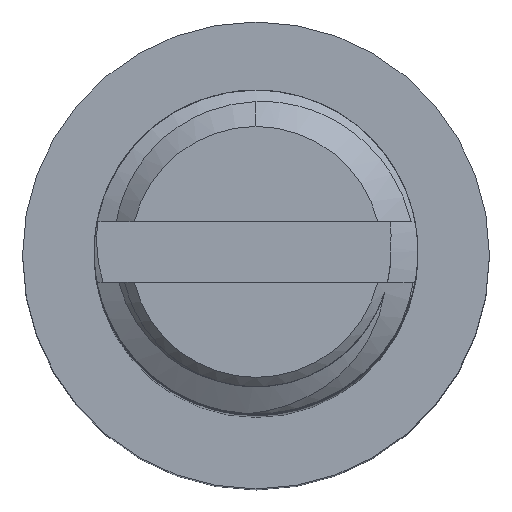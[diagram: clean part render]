
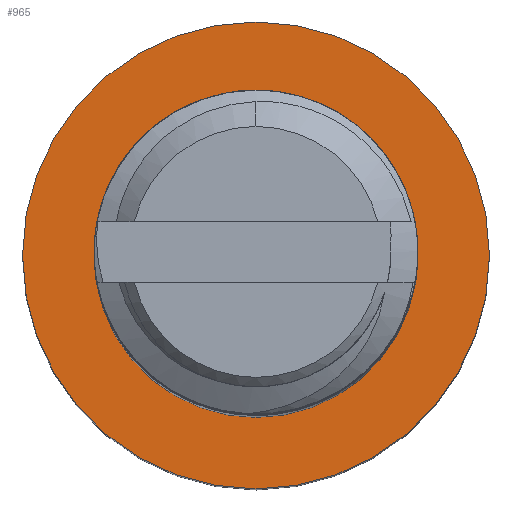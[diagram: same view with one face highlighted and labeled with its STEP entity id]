
A CAD part, top view. The second image highlights one B-rep face of the part: STEP entity #965.
In plain terms, the highlighted planar face has unit normal (0, 0, 1).
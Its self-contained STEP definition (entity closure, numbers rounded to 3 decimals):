
#155 = EDGE_CURVE ( 'NONE', #8737, #4906, #6477, .T. ) ;
#169 = ORIENTED_EDGE ( 'NONE', *, *, #5613, .F. ) ;
#965 = ADVANCED_FACE ( 'NONE', ( #6324, #4373 ), #6561, .T. ) ;
#1108 = CARTESIAN_POINT ( 'NONE',  ( 0., -2.705, -33.528 ) ) ;
#1222 = DIRECTION ( 'NONE',  ( 0., 0., 1. ) ) ;
#1231 = CIRCLE ( 'NONE', #2473, 2.705 ) ;
#1391 = CARTESIAN_POINT ( 'NONE',  ( 0., 0., -33.528 ) ) ;
#1468 = AXIS2_PLACEMENT_3D ( 'NONE', #5819, #2209, #7310 ) ;
#1597 = EDGE_LOOP ( 'NONE', ( #7868, #169 ) ) ;
#2125 = DIRECTION ( 'NONE',  ( 0., 1., 0. ) ) ;
#2209 = DIRECTION ( 'NONE',  ( 0., 0., 1. ) ) ;
#2473 = AXIS2_PLACEMENT_3D ( 'NONE', #7916, #3581, #8627 ) ;
#2607 = CARTESIAN_POINT ( 'NONE',  ( 0., 2.705, -33.528 ) ) ;
#2997 = CIRCLE ( 'NONE', #9325, 3.899 ) ;
#3255 = CARTESIAN_POINT ( 'NONE',  ( 0., 0., -33.528 ) ) ;
#3311 = EDGE_CURVE ( 'NONE', #4906, #8737, #2997, .T. ) ;
#3410 = EDGE_CURVE ( 'NONE', #5366, #4224, #8098, .T. ) ;
#3581 = DIRECTION ( 'NONE',  ( 0., 0., 1. ) ) ;
#4224 = VERTEX_POINT ( 'NONE', #1108 ) ;
#4373 = FACE_BOUND ( 'NONE', #1597, .T. ) ;
#4778 = DIRECTION ( 'NONE',  ( 0., 0., 1. ) ) ;
#4906 = VERTEX_POINT ( 'NONE', #6843 ) ;
#5013 = AXIS2_PLACEMENT_3D ( 'NONE', #3255, #4778, #6480 ) ;
#5366 = VERTEX_POINT ( 'NONE', #2607 ) ;
#5452 = AXIS2_PLACEMENT_3D ( 'NONE', #1391, #6485, #2125 ) ;
#5577 = CARTESIAN_POINT ( 'NONE',  ( 0., 0., -33.528 ) ) ;
#5613 = EDGE_CURVE ( 'NONE', #4224, #5366, #1231, .T. ) ;
#5819 = CARTESIAN_POINT ( 'NONE',  ( 0., 2.705, -33.528 ) ) ;
#6087 = CARTESIAN_POINT ( 'NONE',  ( 0., -3.899, -33.528 ) ) ;
#6318 = DIRECTION ( 'NONE',  ( 0., 1., 0. ) ) ;
#6324 = FACE_OUTER_BOUND ( 'NONE', #7804, .T. ) ;
#6477 = CIRCLE ( 'NONE', #5013, 3.899 ) ;
#6480 = DIRECTION ( 'NONE',  ( 0., 1., 0. ) ) ;
#6485 = DIRECTION ( 'NONE',  ( 0., 0., 1. ) ) ;
#6561 = PLANE ( 'NONE',  #1468 ) ;
#6843 = CARTESIAN_POINT ( 'NONE',  ( 0., 3.899, -33.528 ) ) ;
#7310 = DIRECTION ( 'NONE',  ( 0., -1., 0. ) ) ;
#7804 = EDGE_LOOP ( 'NONE', ( #8370, #8563 ) ) ;
#7868 = ORIENTED_EDGE ( 'NONE', *, *, #3410, .F. ) ;
#7916 = CARTESIAN_POINT ( 'NONE',  ( 0., 0., -33.528 ) ) ;
#8098 = CIRCLE ( 'NONE', #5452, 2.705 ) ;
#8370 = ORIENTED_EDGE ( 'NONE', *, *, #3311, .T. ) ;
#8563 = ORIENTED_EDGE ( 'NONE', *, *, #155, .T. ) ;
#8627 = DIRECTION ( 'NONE',  ( 0., 1., 0. ) ) ;
#8737 = VERTEX_POINT ( 'NONE', #6087 ) ;
#9325 = AXIS2_PLACEMENT_3D ( 'NONE', #5577, #1222, #6318 ) ;
